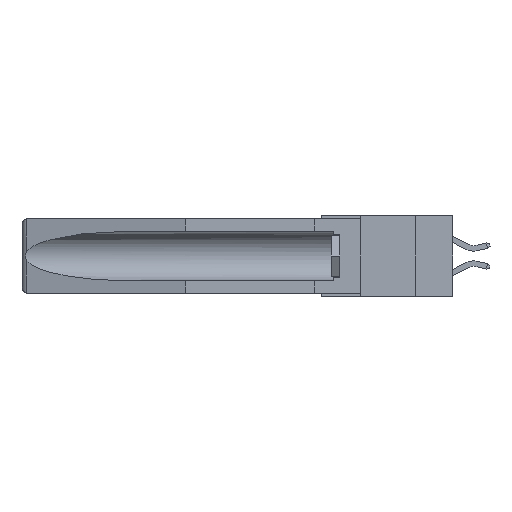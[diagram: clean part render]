
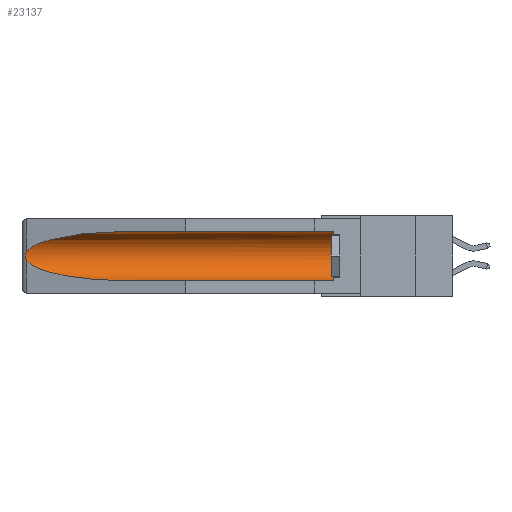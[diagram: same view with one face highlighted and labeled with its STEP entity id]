
A CAD part, left-side view. The second image highlights one B-rep face of the part: STEP entity #23137.
In plain terms, the highlighted cylindrical face has radius 2.857 mm (diameter 5.715 mm), a partial arc.
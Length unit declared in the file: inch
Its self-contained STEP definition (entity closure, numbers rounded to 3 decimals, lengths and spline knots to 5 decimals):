
#754 = DIRECTION ( 'NONE',  ( 0., 0., 1. ) ) ;
#1540 = CIRCLE ( 'NONE', #11598, 0.1125 ) ;
#1580 = CARTESIAN_POINT ( 'NONE',  ( 0.26537, 1.52718, -0.14972 ) ) ;
#2037 = LINE ( 'NONE', #22693, #20298 ) ;
#2056 =( BOUNDED_CURVE ( )  B_SPLINE_CURVE ( 3, ( #5223, #14403, #3082, #20289 ),
 .UNSPECIFIED., .F., .F. ) 
 B_SPLINE_CURVE_WITH_KNOTS ( ( 4, 4 ),
 ( 0.1948, 1.5708 ),
 .UNSPECIFIED. ) 
 CURVE ( )  GEOMETRIC_REPRESENTATION_ITEM ( )  RATIONAL_B_SPLINE_CURVE ( ( 1., 0.848, 0.848, 1. ) ) 
 REPRESENTATION_ITEM ( '' )  );
#2314 = ORIENTED_EDGE ( 'NONE', *, *, #18193, .F. ) ;
#2346 = CARTESIAN_POINT ( 'NONE',  ( 0.155, 1.07973, -0.284 ) ) ;
#3082 = CARTESIAN_POINT ( 'NONE',  ( 0.21114, 1.30732, -0.284 ) ) ;
#3471 = CARTESIAN_POINT ( 'NONE',  ( 0.26654, 1.53092, -0.15636 ) ) ;
#3500 = EDGE_LOOP ( 'NONE', ( #5988, #16144, #11103, #2314, #9938, #5962 ) ) ;
#5223 = CARTESIAN_POINT ( 'NONE',  ( 0.26537, 1.52718, -0.19328 ) ) ;
#5600 = VERTEX_POINT ( 'NONE', #19389 ) ;
#5962 = ORIENTED_EDGE ( 'NONE', *, *, #15970, .T. ) ;
#5988 = ORIENTED_EDGE ( 'NONE', *, *, #9469, .T. ) ;
#6111 = DIRECTION ( 'NONE',  ( 0., 1., 0. ) ) ;
#9211 = CARTESIAN_POINT ( 'NONE',  ( 0.155, -0.30754, -0.059 ) ) ;
#9315 = AXIS2_PLACEMENT_3D ( 'NONE', #9654, #6111, #19107 ) ;
#9469 = EDGE_CURVE ( 'NONE', #5600, #14283, #18966, .T. ) ;
#9511 = VERTEX_POINT ( 'NONE', #2346 ) ;
#9654 = CARTESIAN_POINT ( 'NONE',  ( 0.155, -0.30754, -0.1715 ) ) ;
#9675 = VERTEX_POINT ( 'NONE', #23985 ) ;
#9938 = ORIENTED_EDGE ( 'NONE', *, *, #20059, .T. ) ;
#10175 = CARTESIAN_POINT ( 'NONE',  ( 0.25451, 1.48313, -0.09465 ) ) ;
#10222 = FACE_OUTER_BOUND ( 'NONE', #3500, .T. ) ;
#10584 = VERTEX_POINT ( 'NONE', #22527 ) ;
#10727 = CARTESIAN_POINT ( 'NONE',  ( 0.2675, 1.53308, -0.17534 ) ) ;
#10931 = DIRECTION ( 'NONE',  ( 0., 1., 0. ) ) ;
#11103 = ORIENTED_EDGE ( 'NONE', *, *, #16628, .T. ) ;
#11412 = DIRECTION ( 'NONE',  ( 0., 1., 0. ) ) ;
#11598 = AXIS2_PLACEMENT_3D ( 'NONE', #23657, #13931, #754 ) ;
#11989 = CYLINDRICAL_SURFACE ( 'NONE', #9315, 0.1125 ) ;
#12845 = CARTESIAN_POINT ( 'NONE',  ( 0.2673, 1.53269, -0.17917 ) ) ;
#13241 = EDGE_CURVE ( 'NONE', #14283, #9675, #21509, .T. ) ;
#13332 = VECTOR ( 'NONE', #10931, 39.37008 ) ;
#13931 = DIRECTION ( 'NONE',  ( 0., -1., 0. ) ) ;
#14283 = VERTEX_POINT ( 'NONE', #1580 ) ;
#14403 = CARTESIAN_POINT ( 'NONE',  ( 0.25451, 1.48313, -0.24835 ) ) ;
#15103 = CARTESIAN_POINT ( 'NONE',  ( 0.155, 0.126, -0.059 ) ) ;
#15507 = CARTESIAN_POINT ( 'NONE',  ( 0.155, 1.07973, -0.059 ) ) ;
#15970 = EDGE_CURVE ( 'NONE', #20971, #5600, #18631, .T. ) ;
#16144 = ORIENTED_EDGE ( 'NONE', *, *, #13241, .T. ) ;
#16628 = EDGE_CURVE ( 'NONE', #9675, #9511, #2056, .T. ) ;
#18193 = EDGE_CURVE ( 'NONE', #10584, #9511, #2037, .T. ) ;
#18368 = CARTESIAN_POINT ( 'NONE',  ( 0.26597, 1.5296, -0.19026 ) ) ;
#18631 = LINE ( 'NONE', #9211, #13332 ) ;
#18966 =( BOUNDED_CURVE ( )  B_SPLINE_CURVE ( 3, ( #15507, #21440, #10175, #23342 ),
 .UNSPECIFIED., .F., .F. ) 
 B_SPLINE_CURVE_WITH_KNOTS ( ( 4, 4 ),
 ( 4.71239, 6.08839 ),
 .UNSPECIFIED. ) 
 CURVE ( )  GEOMETRIC_REPRESENTATION_ITEM ( )  RATIONAL_B_SPLINE_CURVE ( ( 1., 0.848, 0.848, 1. ) ) 
 REPRESENTATION_ITEM ( '' )  );
#19107 = DIRECTION ( 'NONE',  ( 0., 0., 1. ) ) ;
#19389 = CARTESIAN_POINT ( 'NONE',  ( 0.155, 1.07973, -0.059 ) ) ;
#20059 = EDGE_CURVE ( 'NONE', #10584, #20971, #1540, .T. ) ;
#20092 = CARTESIAN_POINT ( 'NONE',  ( 0.26597, 1.52961, -0.15275 ) ) ;
#20289 = CARTESIAN_POINT ( 'NONE',  ( 0.155, 1.07973, -0.284 ) ) ;
#20298 = VECTOR ( 'NONE', #11412, 39.37008 ) ;
#20971 = VERTEX_POINT ( 'NONE', #15103 ) ;
#21440 = CARTESIAN_POINT ( 'NONE',  ( 0.21114, 1.30732, -0.059 ) ) ;
#21509 = B_SPLINE_CURVE_WITH_KNOTS ( 'NONE', 3,
 ( #21995, #20092, #3471, #23807, #23961, #10727, #12845, #22160, #18368, #24049 ),
 .UNSPECIFIED., .F., .F.,
 ( 4, 2, 2, 2, 4 ),
 ( 0., 0.00029, 0.00058, 0.00087, 0.00117 ),
 .UNSPECIFIED. ) ;
#21995 = CARTESIAN_POINT ( 'NONE',  ( 0.26537, 1.52718, -0.14972 ) ) ;
#22160 = CARTESIAN_POINT ( 'NONE',  ( 0.26655, 1.53094, -0.18657 ) ) ;
#22527 = CARTESIAN_POINT ( 'NONE',  ( 0.155, 0.126, -0.284 ) ) ;
#22693 = CARTESIAN_POINT ( 'NONE',  ( 0.155, -0.30754, -0.284 ) ) ;
#23137 = ADVANCED_FACE ( 'NONE', ( #10222 ), #11989, .F. ) ;
#23342 = CARTESIAN_POINT ( 'NONE',  ( 0.26537, 1.52718, -0.14972 ) ) ;
#23657 = CARTESIAN_POINT ( 'NONE',  ( 0.155, 0.126, -0.1715 ) ) ;
#23807 = CARTESIAN_POINT ( 'NONE',  ( 0.2673, 1.5327, -0.16383 ) ) ;
#23961 = CARTESIAN_POINT ( 'NONE',  ( 0.2675, 1.53308, -0.16763 ) ) ;
#23985 = CARTESIAN_POINT ( 'NONE',  ( 0.26537, 1.52718, -0.19328 ) ) ;
#24049 = CARTESIAN_POINT ( 'NONE',  ( 0.26537, 1.52718, -0.19328 ) ) ;
